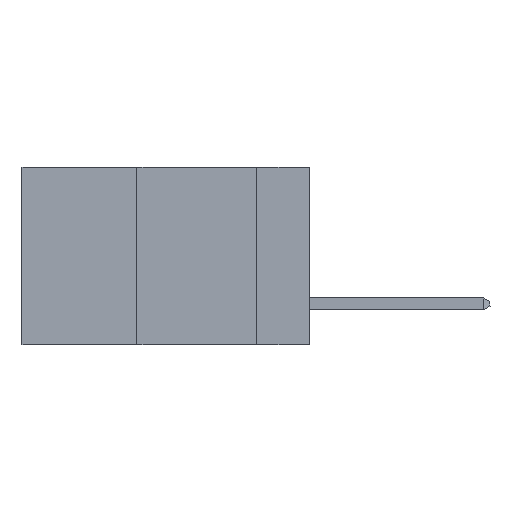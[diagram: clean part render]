
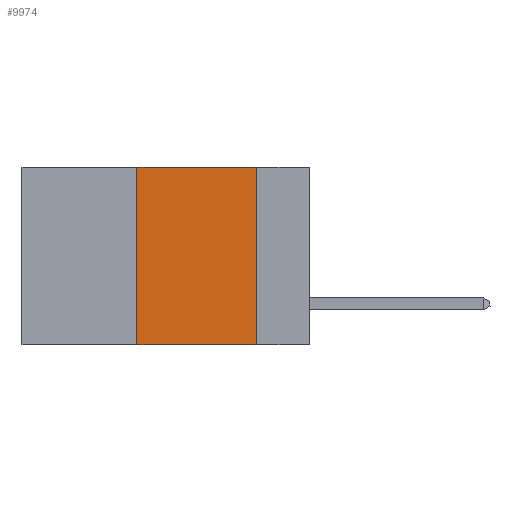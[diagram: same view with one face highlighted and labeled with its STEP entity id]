
A CAD part, left-side view. The second image highlights one B-rep face of the part: STEP entity #9974.
In plain terms, the highlighted planar face has unit normal (-1, 0, 0).
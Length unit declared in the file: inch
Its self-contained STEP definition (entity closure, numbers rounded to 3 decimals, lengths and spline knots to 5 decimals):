
#110 = DIRECTION ( 'NONE',  ( 0., 0., 1. ) ) ;
#876 = LINE ( 'NONE', #3254, #16000 ) ;
#1746 = FACE_OUTER_BOUND ( 'NONE', #14672, .T. ) ;
#2061 = DIRECTION ( 'NONE',  ( 0., 0., -1. ) ) ;
#3254 = CARTESIAN_POINT ( 'NONE',  ( 0., 0.6, 0. ) ) ;
#4219 = LINE ( 'NONE', #10200, #11644 ) ;
#4746 = CARTESIAN_POINT ( 'NONE',  ( 0., 0.11, 0. ) ) ;
#5864 = AXIS2_PLACEMENT_3D ( 'NONE', #15189, #11060, #2061 ) ;
#6132 = VERTEX_POINT ( 'NONE', #10872 ) ;
#6957 = LINE ( 'NONE', #17552, #17726 ) ;
#7211 = VERTEX_POINT ( 'NONE', #8743 ) ;
#7708 = DIRECTION ( 'NONE',  ( 0., 0., -1. ) ) ;
#7955 = VECTOR ( 'NONE', #7708, 39.37008 ) ;
#8173 = ORIENTED_EDGE ( 'NONE', *, *, #13882, .F. ) ;
#8743 = CARTESIAN_POINT ( 'NONE',  ( 0., 0.36, -0.37 ) ) ;
#8969 = EDGE_CURVE ( 'NONE', #7211, #6132, #4219, .T. ) ;
#9602 = PLANE ( 'NONE',  #5864 ) ;
#9974 = ADVANCED_FACE ( 'NONE', ( #1746 ), #9602, .F. ) ;
#10200 = CARTESIAN_POINT ( 'NONE',  ( 0., 0.6, -0.37 ) ) ;
#10872 = CARTESIAN_POINT ( 'NONE',  ( 0., 0.11, -0.37 ) ) ;
#11060 = DIRECTION ( 'NONE',  ( 1., 0., 0. ) ) ;
#11644 = VECTOR ( 'NONE', #18469, 39.37008 ) ;
#12035 = CARTESIAN_POINT ( 'NONE',  ( 0., 0.11, 0. ) ) ;
#12268 = LINE ( 'NONE', #12035, #7955 ) ;
#12438 = ORIENTED_EDGE ( 'NONE', *, *, #8969, .T. ) ;
#13080 = ORIENTED_EDGE ( 'NONE', *, *, #17849, .F. ) ;
#13526 = ORIENTED_EDGE ( 'NONE', *, *, #15952, .F. ) ;
#13551 = DIRECTION ( 'NONE',  ( 0., -1., 0. ) ) ;
#13882 = EDGE_CURVE ( 'NONE', #14231, #14893, #876, .T. ) ;
#14231 = VERTEX_POINT ( 'NONE', #18386 ) ;
#14672 = EDGE_LOOP ( 'NONE', ( #13526, #8173, #13080, #12438 ) ) ;
#14893 = VERTEX_POINT ( 'NONE', #4746 ) ;
#15189 = CARTESIAN_POINT ( 'NONE',  ( 0., 0.6, 0. ) ) ;
#15952 = EDGE_CURVE ( 'NONE', #14893, #6132, #12268, .T. ) ;
#16000 = VECTOR ( 'NONE', #13551, 39.37008 ) ;
#17552 = CARTESIAN_POINT ( 'NONE',  ( 0., 0.36, 0. ) ) ;
#17726 = VECTOR ( 'NONE', #110, 39.37008 ) ;
#17849 = EDGE_CURVE ( 'NONE', #7211, #14231, #6957, .T. ) ;
#18386 = CARTESIAN_POINT ( 'NONE',  ( 0., 0.36, 0. ) ) ;
#18469 = DIRECTION ( 'NONE',  ( 0., -1., 0. ) ) ;
